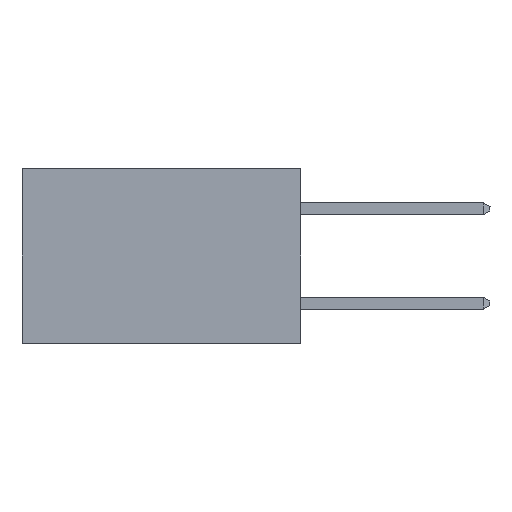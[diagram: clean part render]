
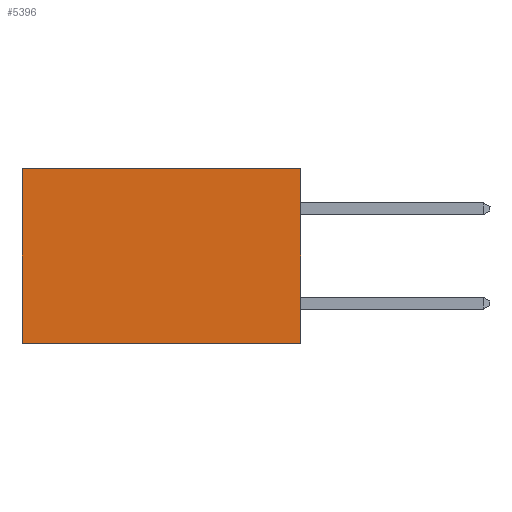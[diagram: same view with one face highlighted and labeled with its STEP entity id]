
A CAD part, left-side view. The second image highlights one B-rep face of the part: STEP entity #5396.
In plain terms, the highlighted planar face has unit normal (-1, 0, 0).
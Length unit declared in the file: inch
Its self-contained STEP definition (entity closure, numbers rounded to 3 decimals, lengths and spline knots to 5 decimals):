
#85 = DIRECTION ( 'NONE',  ( 0., 1., 0. ) ) ;
#499 = LINE ( 'NONE', #7304, #791 ) ;
#785 = EDGE_CURVE ( 'NONE', #12112, #4597, #8162, .T. ) ;
#791 = VECTOR ( 'NONE', #7310, 39.37008 ) ;
#1191 = EDGE_CURVE ( 'NONE', #5819, #2705, #11570, .T. ) ;
#1361 = CARTESIAN_POINT ( 'NONE',  ( 0.277, 0.59, -0.37 ) ) ;
#2036 = LINE ( 'NONE', #6794, #6598 ) ;
#2705 = VERTEX_POINT ( 'NONE', #7556 ) ;
#3144 = CARTESIAN_POINT ( 'NONE',  ( 0.277, 0., -0.37 ) ) ;
#3215 = CARTESIAN_POINT ( 'NONE',  ( 0.277, 0., 0. ) ) ;
#3441 = AXIS2_PLACEMENT_3D ( 'NONE', #11503, #10124, #9862 ) ;
#3970 = VECTOR ( 'NONE', #8788, 39.37008 ) ;
#4597 = VERTEX_POINT ( 'NONE', #12209 ) ;
#4720 = FACE_OUTER_BOUND ( 'NONE', #8050, .T. ) ;
#5396 = ADVANCED_FACE ( 'NONE', ( #4720 ), #9501, .F. ) ;
#5612 = VECTOR ( 'NONE', #10251, 39.37008 ) ;
#5819 = VERTEX_POINT ( 'NONE', #8086 ) ;
#5996 = ORIENTED_EDGE ( 'NONE', *, *, #1191, .T. ) ;
#6598 = VECTOR ( 'NONE', #85, 39.37008 ) ;
#6794 = CARTESIAN_POINT ( 'NONE',  ( 0.277, 0., 0. ) ) ;
#7036 = EDGE_CURVE ( 'NONE', #4597, #2705, #499, .T. ) ;
#7304 = CARTESIAN_POINT ( 'NONE',  ( 0.277, 0., -0.37 ) ) ;
#7310 = DIRECTION ( 'NONE',  ( 0., 1., 0. ) ) ;
#7556 = CARTESIAN_POINT ( 'NONE',  ( 0.277, 0.59, -0.37 ) ) ;
#8050 = EDGE_LOOP ( 'NONE', ( #5996, #10589, #10487, #8362 ) ) ;
#8086 = CARTESIAN_POINT ( 'NONE',  ( 0.277, 0.59, 0. ) ) ;
#8162 = LINE ( 'NONE', #3144, #5612 ) ;
#8362 = ORIENTED_EDGE ( 'NONE', *, *, #10321, .T. ) ;
#8788 = DIRECTION ( 'NONE',  ( 0., 0., -1. ) ) ;
#9501 = PLANE ( 'NONE',  #3441 ) ;
#9862 = DIRECTION ( 'NONE',  ( 0., 0., -1. ) ) ;
#10124 = DIRECTION ( 'NONE',  ( 1., 0., 0. ) ) ;
#10251 = DIRECTION ( 'NONE',  ( 0., 0., -1. ) ) ;
#10321 = EDGE_CURVE ( 'NONE', #12112, #5819, #2036, .T. ) ;
#10487 = ORIENTED_EDGE ( 'NONE', *, *, #785, .F. ) ;
#10589 = ORIENTED_EDGE ( 'NONE', *, *, #7036, .F. ) ;
#11503 = CARTESIAN_POINT ( 'NONE',  ( 0.277, 0., -0.37 ) ) ;
#11570 = LINE ( 'NONE', #1361, #3970 ) ;
#12112 = VERTEX_POINT ( 'NONE', #3215 ) ;
#12209 = CARTESIAN_POINT ( 'NONE',  ( 0.277, 0., -0.37 ) ) ;
